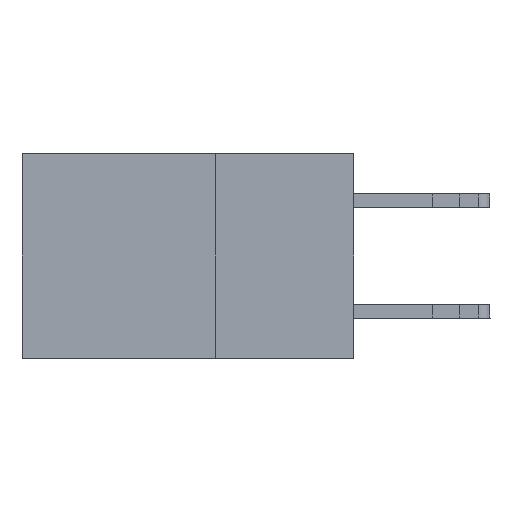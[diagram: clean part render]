
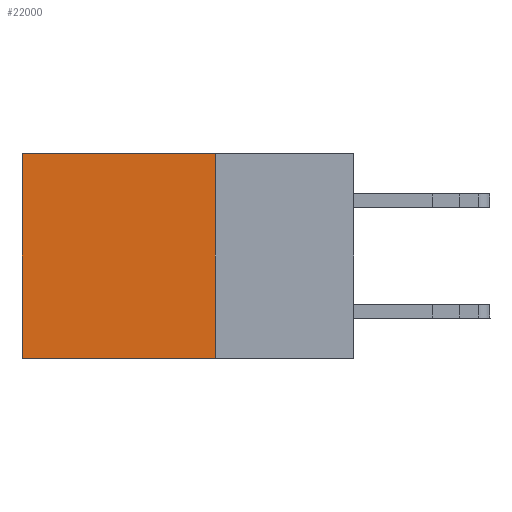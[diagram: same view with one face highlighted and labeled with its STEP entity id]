
A CAD part, left-side view. The second image highlights one B-rep face of the part: STEP entity #22000.
In plain terms, the highlighted planar face has unit normal (-1, 0, 0).
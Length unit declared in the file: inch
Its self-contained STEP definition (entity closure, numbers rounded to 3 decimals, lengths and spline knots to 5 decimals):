
#870 = EDGE_CURVE ( 'NONE', #6845, #20153, #14119, .T. ) ;
#1529 = EDGE_CURVE ( 'NONE', #6845, #32064, #2480, .T. ) ;
#2480 = LINE ( 'NONE', #12577, #28057 ) ;
#2704 = EDGE_CURVE ( 'NONE', #32064, #9181, #28608, .T. ) ;
#5967 = ORIENTED_EDGE ( 'NONE', *, *, #870, .F. ) ;
#6038 = CARTESIAN_POINT ( 'NONE',  ( 0.2875, 0.6, -0.37 ) ) ;
#6845 = VERTEX_POINT ( 'NONE', #11390 ) ;
#7604 = DIRECTION ( 'NONE',  ( 0., 0., -1. ) ) ;
#9181 = VERTEX_POINT ( 'NONE', #6038 ) ;
#11390 = CARTESIAN_POINT ( 'NONE',  ( 0.2875, 0.25, 0. ) ) ;
#11635 = DIRECTION ( 'NONE',  ( 0., 0., -1. ) ) ;
#12577 = CARTESIAN_POINT ( 'NONE',  ( 0.2875, 0.25, 0. ) ) ;
#12670 = ORIENTED_EDGE ( 'NONE', *, *, #21714, .F. ) ;
#13683 = CARTESIAN_POINT ( 'NONE',  ( 0.2875, 0.25, -0.37 ) ) ;
#14119 = LINE ( 'NONE', #21728, #23793 ) ;
#15230 = DIRECTION ( 'NONE',  ( 1., 0., 0. ) ) ;
#15634 = ORIENTED_EDGE ( 'NONE', *, *, #1529, .T. ) ;
#16043 = DIRECTION ( 'NONE',  ( 0., 0., -1. ) ) ;
#16336 = CARTESIAN_POINT ( 'NONE',  ( 0.2875, 0.6, 0. ) ) ;
#16510 = CARTESIAN_POINT ( 'NONE',  ( 0.2875, 0.25, -0.37 ) ) ;
#18199 = CARTESIAN_POINT ( 'NONE',  ( 0.2875, 0.6, 0. ) ) ;
#19868 = AXIS2_PLACEMENT_3D ( 'NONE', #32589, #15230, #7604 ) ;
#20153 = VERTEX_POINT ( 'NONE', #13683 ) ;
#21054 = EDGE_LOOP ( 'NONE', ( #25503, #12670, #5967, #15634 ) ) ;
#21714 = EDGE_CURVE ( 'NONE', #20153, #9181, #21790, .T. ) ;
#21728 = CARTESIAN_POINT ( 'NONE',  ( 0.2875, 0.25, 0. ) ) ;
#21790 = LINE ( 'NONE', #16510, #28290 ) ;
#22000 = ADVANCED_FACE ( 'NONE', ( #32423 ), #22489, .F. ) ;
#22489 = PLANE ( 'NONE',  #19868 ) ;
#22659 = DIRECTION ( 'NONE',  ( 0., 1., 0. ) ) ;
#23793 = VECTOR ( 'NONE', #11635, 39.37008 ) ;
#25503 = ORIENTED_EDGE ( 'NONE', *, *, #2704, .T. ) ;
#28057 = VECTOR ( 'NONE', #22659, 39.37008 ) ;
#28290 = VECTOR ( 'NONE', #32209, 39.37008 ) ;
#28418 = VECTOR ( 'NONE', #16043, 39.37008 ) ;
#28608 = LINE ( 'NONE', #18199, #28418 ) ;
#32064 = VERTEX_POINT ( 'NONE', #16336 ) ;
#32209 = DIRECTION ( 'NONE',  ( 0., 1., 0. ) ) ;
#32423 = FACE_OUTER_BOUND ( 'NONE', #21054, .T. ) ;
#32589 = CARTESIAN_POINT ( 'NONE',  ( 0.2875, 0.25, 0. ) ) ;
